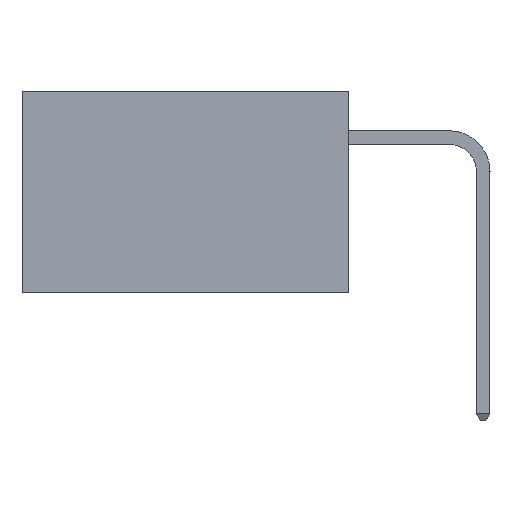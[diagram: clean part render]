
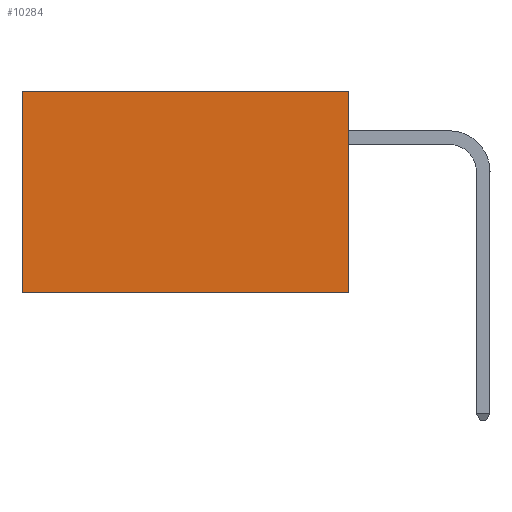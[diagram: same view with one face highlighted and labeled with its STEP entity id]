
A CAD part, left-side view. The second image highlights one B-rep face of the part: STEP entity #10284.
In plain terms, the highlighted planar face has unit normal (-1, 0, 0).
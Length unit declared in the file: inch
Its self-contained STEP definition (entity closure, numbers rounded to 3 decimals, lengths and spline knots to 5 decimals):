
#132 = EDGE_CURVE ( 'NONE', #9742, #6539, #5685, .T. ) ;
#932 = VECTOR ( 'NONE', #8160, 39.37008 ) ;
#2177 = PLANE ( 'NONE',  #10303 ) ;
#2461 = EDGE_CURVE ( 'NONE', #13736, #2590, #13563, .T. ) ;
#2518 = VECTOR ( 'NONE', #9835, 39.37008 ) ;
#2577 = CARTESIAN_POINT ( 'NONE',  ( 0.2875, 0., 0. ) ) ;
#2590 = VERTEX_POINT ( 'NONE', #2840 ) ;
#2840 = CARTESIAN_POINT ( 'NONE',  ( 0.2875, 0.6, -0.37 ) ) ;
#3305 = CARTESIAN_POINT ( 'NONE',  ( 0.2875, 0., 0. ) ) ;
#3352 = DIRECTION ( 'NONE',  ( 0., 0., -1. ) ) ;
#3667 = CARTESIAN_POINT ( 'NONE',  ( 0.2875, 0., 0. ) ) ;
#3873 = ORIENTED_EDGE ( 'NONE', *, *, #5854, .T. ) ;
#4135 = LINE ( 'NONE', #14130, #13211 ) ;
#5043 = DIRECTION ( 'NONE',  ( 0., 0., -1. ) ) ;
#5685 = LINE ( 'NONE', #2577, #2518 ) ;
#5724 = CARTESIAN_POINT ( 'NONE',  ( 0.2875, 0., -0.37 ) ) ;
#5854 = EDGE_CURVE ( 'NONE', #6539, #2590, #4135, .T. ) ;
#6539 = VERTEX_POINT ( 'NONE', #14917 ) ;
#7088 = VECTOR ( 'NONE', #5043, 39.37008 ) ;
#7304 = EDGE_LOOP ( 'NONE', ( #3873, #10965, #11635, #10842 ) ) ;
#7670 = CARTESIAN_POINT ( 'NONE',  ( 0.2875, 0., -0.37 ) ) ;
#8160 = DIRECTION ( 'NONE',  ( 0., 1., 0. ) ) ;
#8694 = EDGE_CURVE ( 'NONE', #9742, #13736, #13296, .T. ) ;
#9742 = VERTEX_POINT ( 'NONE', #3667 ) ;
#9835 = DIRECTION ( 'NONE',  ( 0., 1., 0. ) ) ;
#10283 = DIRECTION ( 'NONE',  ( 0., 0., -1. ) ) ;
#10284 = ADVANCED_FACE ( 'NONE', ( #14624 ), #2177, .F. ) ;
#10303 = AXIS2_PLACEMENT_3D ( 'NONE', #3305, #10517, #3352 ) ;
#10517 = DIRECTION ( 'NONE',  ( 1., 0., 0. ) ) ;
#10842 = ORIENTED_EDGE ( 'NONE', *, *, #132, .T. ) ;
#10965 = ORIENTED_EDGE ( 'NONE', *, *, #2461, .F. ) ;
#11635 = ORIENTED_EDGE ( 'NONE', *, *, #8694, .F. ) ;
#13211 = VECTOR ( 'NONE', #10283, 39.37008 ) ;
#13296 = LINE ( 'NONE', #13329, #7088 ) ;
#13329 = CARTESIAN_POINT ( 'NONE',  ( 0.2875, 0., 0. ) ) ;
#13563 = LINE ( 'NONE', #5724, #932 ) ;
#13736 = VERTEX_POINT ( 'NONE', #7670 ) ;
#14130 = CARTESIAN_POINT ( 'NONE',  ( 0.2875, 0.6, 0. ) ) ;
#14624 = FACE_OUTER_BOUND ( 'NONE', #7304, .T. ) ;
#14917 = CARTESIAN_POINT ( 'NONE',  ( 0.2875, 0.6, 0. ) ) ;
